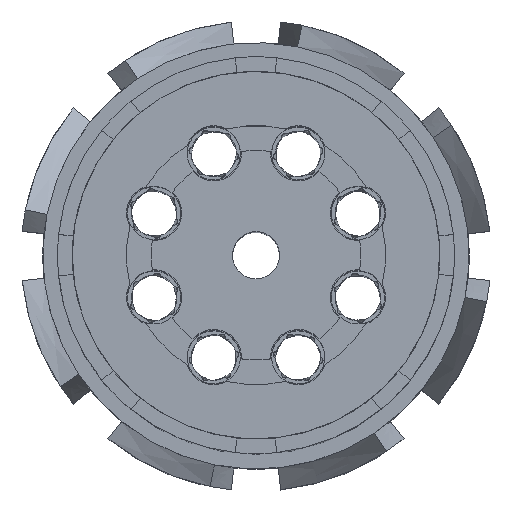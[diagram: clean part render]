
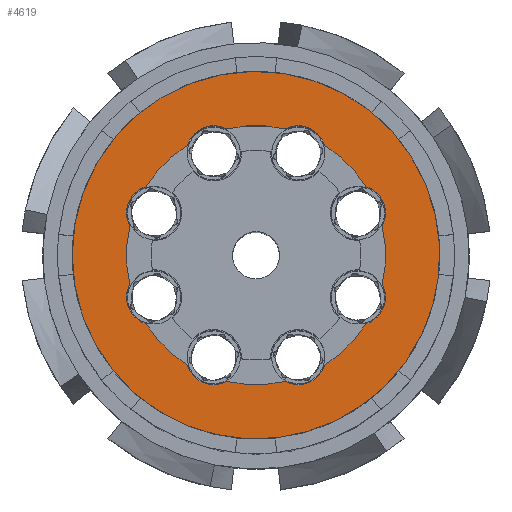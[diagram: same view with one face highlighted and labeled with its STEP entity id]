
A CAD part, top view. The second image highlights one B-rep face of the part: STEP entity #4619.
In plain terms, the highlighted face is planar.
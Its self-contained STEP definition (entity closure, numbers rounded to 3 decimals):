
#4432=CARTESIAN_POINT('',(10.248,35.5,-14.339));
#4433=VERTEX_POINT('',#4432);
#4449=CARTESIAN_POINT('',(14.339,35.5,-10.248));
#4450=VERTEX_POINT('',#4449);
#4457=CARTESIAN_POINT('',(10.607,35.5,-10.607));
#4458=DIRECTION('',(0.0,-1.0,0.0));
#4459=DIRECTION('',(1.0,0.0,0.0));
#4460=AXIS2_PLACEMENT_3D('',#4457,#4458,#4459);
#4461=CIRCLE('',#4460,3.75);
#4462=EDGE_CURVE('',#4433,#4450,#4461,.T.);
#4467=CARTESIAN_POINT('',(0.0,35.5,0.0));
#4468=DIRECTION('',(0.0,-1.0,0.0));
#4469=DIRECTION('',(0.0,0.0,-1.0));
#4470=AXIS2_PLACEMENT_3D('',#4467,#4468,#4469);
#4471=PLANE('',#4470);
#4472=CARTESIAN_POINT('',(25.0,35.5,0.));
#4473=VERTEX_POINT('',#4472);
#4474=CARTESIAN_POINT('',(0.0,35.5,0.0));
#4475=DIRECTION('',(0.0,-1.0,0.0));
#4476=DIRECTION('',(-1.0,0.0,0.0));
#4477=AXIS2_PLACEMENT_3D('',#4474,#4475,#4476);
#4478=CIRCLE('',#4477,25.0);
#4479=EDGE_CURVE('',#4473,#4473,#4478,.T.);
#4480=ORIENTED_EDGE('',*,*,#4479,.F.);
#4481=EDGE_LOOP('',(#4480));
#4482=FACE_OUTER_BOUND('',#4481,.T.);
#4483=ORIENTED_EDGE('',*,*,#4462,.T.);
#4484=CARTESIAN_POINT('',(17.386,35.5,-2.893));
#4485=VERTEX_POINT('',#4484);
#4486=CARTESIAN_POINT('',(0.0,35.5,0.0));
#4487=DIRECTION('',(0.0,-1.0,0.0));
#4488=DIRECTION('',(0.986,0.0,-0.164));
#4489=AXIS2_PLACEMENT_3D('',#4486,#4487,#4488);
#4490=CIRCLE('',#4489,17.625);
#4491=EDGE_CURVE('',#4450,#4485,#4490,.T.);
#4492=ORIENTED_EDGE('',*,*,#4491,.T.);
#4493=CARTESIAN_POINT('',(17.386,35.5,2.893));
#4494=VERTEX_POINT('',#4493);
#4495=CARTESIAN_POINT('',(15.0,35.5,0.));
#4496=DIRECTION('',(0.0,-1.0,0.0));
#4497=DIRECTION('',(1.0,0.0,0.0));
#4498=AXIS2_PLACEMENT_3D('',#4495,#4496,#4497);
#4499=CIRCLE('',#4498,3.75);
#4500=EDGE_CURVE('',#4485,#4494,#4499,.T.);
#4501=ORIENTED_EDGE('',*,*,#4500,.T.);
#4502=CARTESIAN_POINT('',(14.339,35.5,10.248));
#4503=VERTEX_POINT('',#4502);
#4504=CARTESIAN_POINT('',(0.0,35.5,0.0));
#4505=DIRECTION('',(0.0,-1.0,0.0));
#4506=DIRECTION('',(0.814,0.0,0.581));
#4507=AXIS2_PLACEMENT_3D('',#4504,#4505,#4506);
#4508=CIRCLE('',#4507,17.625);
#4509=EDGE_CURVE('',#4494,#4503,#4508,.T.);
#4510=ORIENTED_EDGE('',*,*,#4509,.T.);
#4511=CARTESIAN_POINT('',(10.248,35.5,14.339));
#4512=VERTEX_POINT('',#4511);
#4513=CARTESIAN_POINT('',(10.607,35.5,10.607));
#4514=DIRECTION('',(0.0,-1.0,0.0));
#4515=DIRECTION('',(1.0,0.0,0.0));
#4516=AXIS2_PLACEMENT_3D('',#4513,#4514,#4515);
#4517=CIRCLE('',#4516,3.75);
#4518=EDGE_CURVE('',#4503,#4512,#4517,.T.);
#4519=ORIENTED_EDGE('',*,*,#4518,.T.);
#4520=CARTESIAN_POINT('',(2.893,35.5,17.386));
#4521=VERTEX_POINT('',#4520);
#4522=CARTESIAN_POINT('',(0.0,35.5,0.0));
#4523=DIRECTION('',(0.0,-1.0,0.0));
#4524=DIRECTION('',(0.164,0.0,0.986));
#4525=AXIS2_PLACEMENT_3D('',#4522,#4523,#4524);
#4526=CIRCLE('',#4525,17.625);
#4527=EDGE_CURVE('',#4512,#4521,#4526,.T.);
#4528=ORIENTED_EDGE('',*,*,#4527,.T.);
#4529=CARTESIAN_POINT('',(-2.893,35.5,17.386));
#4530=VERTEX_POINT('',#4529);
#4531=CARTESIAN_POINT('',(0.,35.5,15.0));
#4532=DIRECTION('',(0.0,-1.0,0.0));
#4533=DIRECTION('',(1.0,0.0,0.0));
#4534=AXIS2_PLACEMENT_3D('',#4531,#4532,#4533);
#4535=CIRCLE('',#4534,3.75);
#4536=EDGE_CURVE('',#4521,#4530,#4535,.T.);
#4537=ORIENTED_EDGE('',*,*,#4536,.T.);
#4538=CARTESIAN_POINT('',(-10.248,35.5,14.339));
#4539=VERTEX_POINT('',#4538);
#4540=CARTESIAN_POINT('',(0.0,35.5,0.0));
#4541=DIRECTION('',(0.0,-1.0,0.0));
#4542=DIRECTION('',(-0.581,0.0,0.814));
#4543=AXIS2_PLACEMENT_3D('',#4540,#4541,#4542);
#4544=CIRCLE('',#4543,17.625);
#4545=EDGE_CURVE('',#4530,#4539,#4544,.T.);
#4546=ORIENTED_EDGE('',*,*,#4545,.T.);
#4547=CARTESIAN_POINT('',(-14.339,35.5,10.248));
#4548=VERTEX_POINT('',#4547);
#4549=CARTESIAN_POINT('',(-10.607,35.5,10.607));
#4550=DIRECTION('',(0.0,-1.0,0.0));
#4551=DIRECTION('',(1.0,0.0,0.0));
#4552=AXIS2_PLACEMENT_3D('',#4549,#4550,#4551);
#4553=CIRCLE('',#4552,3.75);
#4554=EDGE_CURVE('',#4539,#4548,#4553,.T.);
#4555=ORIENTED_EDGE('',*,*,#4554,.T.);
#4556=CARTESIAN_POINT('',(-17.386,35.5,2.893));
#4557=VERTEX_POINT('',#4556);
#4558=CARTESIAN_POINT('',(0.0,35.5,0.0));
#4559=DIRECTION('',(0.0,-1.0,0.0));
#4560=DIRECTION('',(-0.986,0.0,0.164));
#4561=AXIS2_PLACEMENT_3D('',#4558,#4559,#4560);
#4562=CIRCLE('',#4561,17.625);
#4563=EDGE_CURVE('',#4548,#4557,#4562,.T.);
#4564=ORIENTED_EDGE('',*,*,#4563,.T.);
#4565=CARTESIAN_POINT('',(-17.386,35.5,-2.893));
#4566=VERTEX_POINT('',#4565);
#4567=CARTESIAN_POINT('',(-15.0,35.5,0.));
#4568=DIRECTION('',(0.0,-1.0,0.0));
#4569=DIRECTION('',(1.0,0.0,0.0));
#4570=AXIS2_PLACEMENT_3D('',#4567,#4568,#4569);
#4571=CIRCLE('',#4570,3.75);
#4572=EDGE_CURVE('',#4557,#4566,#4571,.T.);
#4573=ORIENTED_EDGE('',*,*,#4572,.T.);
#4574=CARTESIAN_POINT('',(-14.339,35.5,-10.248));
#4575=VERTEX_POINT('',#4574);
#4576=CARTESIAN_POINT('',(0.0,35.5,0.0));
#4577=DIRECTION('',(0.0,-1.0,0.0));
#4578=DIRECTION('',(-0.814,0.0,-0.581));
#4579=AXIS2_PLACEMENT_3D('',#4576,#4577,#4578);
#4580=CIRCLE('',#4579,17.625);
#4581=EDGE_CURVE('',#4566,#4575,#4580,.T.);
#4582=ORIENTED_EDGE('',*,*,#4581,.T.);
#4583=CARTESIAN_POINT('',(-10.248,35.5,-14.339));
#4584=VERTEX_POINT('',#4583);
#4585=CARTESIAN_POINT('',(-10.607,35.5,-10.607));
#4586=DIRECTION('',(0.0,-1.0,0.0));
#4587=DIRECTION('',(1.0,0.0,0.0));
#4588=AXIS2_PLACEMENT_3D('',#4585,#4586,#4587);
#4589=CIRCLE('',#4588,3.75);
#4590=EDGE_CURVE('',#4575,#4584,#4589,.T.);
#4591=ORIENTED_EDGE('',*,*,#4590,.T.);
#4592=CARTESIAN_POINT('',(-2.893,35.5,-17.386));
#4593=VERTEX_POINT('',#4592);
#4594=CARTESIAN_POINT('',(0.0,35.5,0.0));
#4595=DIRECTION('',(0.0,-1.0,0.0));
#4596=DIRECTION('',(-0.164,0.0,-0.986));
#4597=AXIS2_PLACEMENT_3D('',#4594,#4595,#4596);
#4598=CIRCLE('',#4597,17.625);
#4599=EDGE_CURVE('',#4584,#4593,#4598,.T.);
#4600=ORIENTED_EDGE('',*,*,#4599,.T.);
#4601=CARTESIAN_POINT('',(2.893,35.5,-17.386));
#4602=VERTEX_POINT('',#4601);
#4603=CARTESIAN_POINT('',(0.,35.5,-15.0));
#4604=DIRECTION('',(0.0,-1.0,0.0));
#4605=DIRECTION('',(1.0,0.0,0.0));
#4606=AXIS2_PLACEMENT_3D('',#4603,#4604,#4605);
#4607=CIRCLE('',#4606,3.75);
#4608=EDGE_CURVE('',#4593,#4602,#4607,.T.);
#4609=ORIENTED_EDGE('',*,*,#4608,.T.);
#4610=CARTESIAN_POINT('',(0.0,35.5,0.0));
#4611=DIRECTION('',(0.0,-1.0,0.0));
#4612=DIRECTION('',(0.581,0.0,-0.814));
#4613=AXIS2_PLACEMENT_3D('',#4610,#4611,#4612);
#4614=CIRCLE('',#4613,17.625);
#4615=EDGE_CURVE('',#4602,#4433,#4614,.T.);
#4616=ORIENTED_EDGE('',*,*,#4615,.T.);
#4617=EDGE_LOOP('',(#4483,#4492,#4501,#4510,#4519,#4528,#4537,#4546,#4555,#4564,#4573,#4582,#4591,#4600,#4609,#4616));
#4618=FACE_BOUND('',#4617,.T.);
#4619=ADVANCED_FACE('',(#4482,#4618),#4471,.F.);
